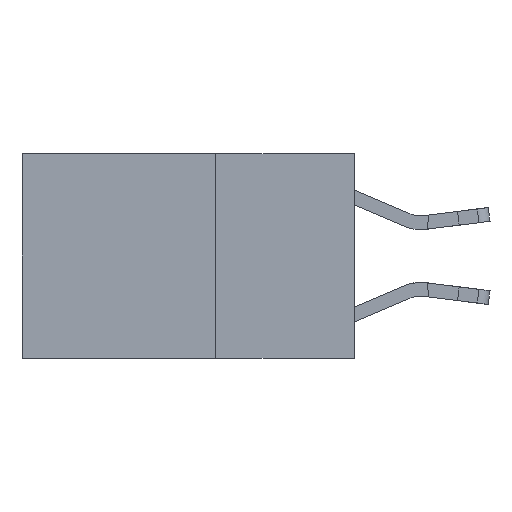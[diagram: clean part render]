
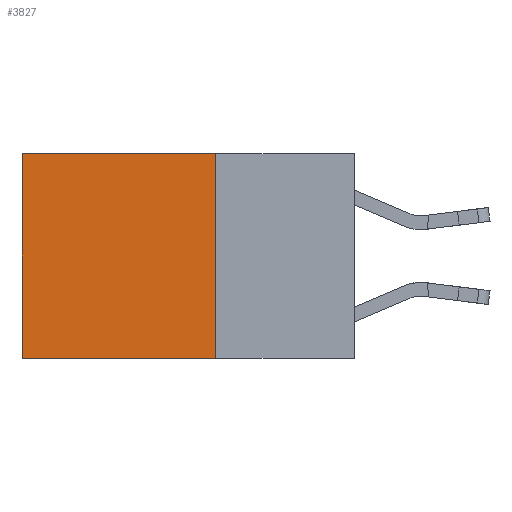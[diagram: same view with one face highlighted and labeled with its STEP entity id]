
A CAD part, left-side view. The second image highlights one B-rep face of the part: STEP entity #3827.
In plain terms, the highlighted planar face has unit normal (-1, 0, 0).
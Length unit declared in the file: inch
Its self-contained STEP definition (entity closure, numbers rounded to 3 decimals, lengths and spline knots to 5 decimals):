
#166 = LINE ( 'NONE', #2234, #4345 ) ;
#457 = LINE ( 'NONE', #8141, #14392 ) ;
#458 = VECTOR ( 'NONE', #6617, 39.37008 ) ;
#495 = DIRECTION ( 'NONE',  ( 0., 1., 0. ) ) ;
#779 = DIRECTION ( 'NONE',  ( 1., 0., 0. ) ) ;
#933 = CARTESIAN_POINT ( 'NONE',  ( 0.2625, 0.25, 0. ) ) ;
#2120 = VERTEX_POINT ( 'NONE', #11618 ) ;
#2234 = CARTESIAN_POINT ( 'NONE',  ( 0.2625, 0.25, 0. ) ) ;
#3827 = ADVANCED_FACE ( 'NONE', ( #16284 ), #16365, .F. ) ;
#3972 = LINE ( 'NONE', #7889, #458 ) ;
#4067 = AXIS2_PLACEMENT_3D ( 'NONE', #7510, #779, #6151 ) ;
#4345 = VECTOR ( 'NONE', #12649, 39.37008 ) ;
#4978 = VERTEX_POINT ( 'NONE', #16202 ) ;
#5642 = VERTEX_POINT ( 'NONE', #933 ) ;
#6151 = DIRECTION ( 'NONE',  ( 0., 0., -1. ) ) ;
#6617 = DIRECTION ( 'NONE',  ( 0., 0., -1. ) ) ;
#6952 = DIRECTION ( 'NONE',  ( 0., 1., 0. ) ) ;
#7272 = ORIENTED_EDGE ( 'NONE', *, *, #10042, .T. ) ;
#7510 = CARTESIAN_POINT ( 'NONE',  ( 0.2625, 0.25, 0. ) ) ;
#7889 = CARTESIAN_POINT ( 'NONE',  ( 0.2625, 0.6, 0. ) ) ;
#8141 = CARTESIAN_POINT ( 'NONE',  ( 0.2625, 0.25, -0.37 ) ) ;
#10042 = EDGE_CURVE ( 'NONE', #15126, #2120, #3972, .T. ) ;
#10078 = ORIENTED_EDGE ( 'NONE', *, *, #14088, .F. ) ;
#10551 = ORIENTED_EDGE ( 'NONE', *, *, #14371, .F. ) ;
#10630 = LINE ( 'NONE', #12276, #14372 ) ;
#11618 = CARTESIAN_POINT ( 'NONE',  ( 0.2625, 0.6, -0.37 ) ) ;
#12276 = CARTESIAN_POINT ( 'NONE',  ( 0.2625, 0.25, 0. ) ) ;
#12649 = DIRECTION ( 'NONE',  ( 0., 0., -1. ) ) ;
#13180 = EDGE_CURVE ( 'NONE', #5642, #15126, #10630, .T. ) ;
#13984 = ORIENTED_EDGE ( 'NONE', *, *, #13180, .T. ) ;
#14088 = EDGE_CURVE ( 'NONE', #4978, #2120, #457, .T. ) ;
#14371 = EDGE_CURVE ( 'NONE', #5642, #4978, #166, .T. ) ;
#14372 = VECTOR ( 'NONE', #495, 39.37008 ) ;
#14392 = VECTOR ( 'NONE', #6952, 39.37008 ) ;
#14956 = EDGE_LOOP ( 'NONE', ( #7272, #10078, #10551, #13984 ) ) ;
#15126 = VERTEX_POINT ( 'NONE', #15811 ) ;
#15811 = CARTESIAN_POINT ( 'NONE',  ( 0.2625, 0.6, 0. ) ) ;
#16202 = CARTESIAN_POINT ( 'NONE',  ( 0.2625, 0.25, -0.37 ) ) ;
#16284 = FACE_OUTER_BOUND ( 'NONE', #14956, .T. ) ;
#16365 = PLANE ( 'NONE',  #4067 ) ;
